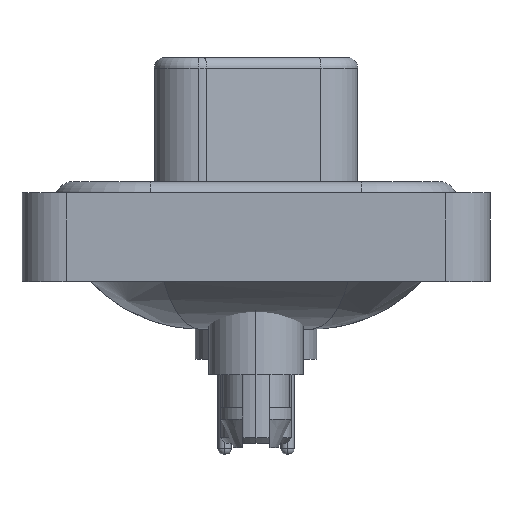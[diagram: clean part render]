
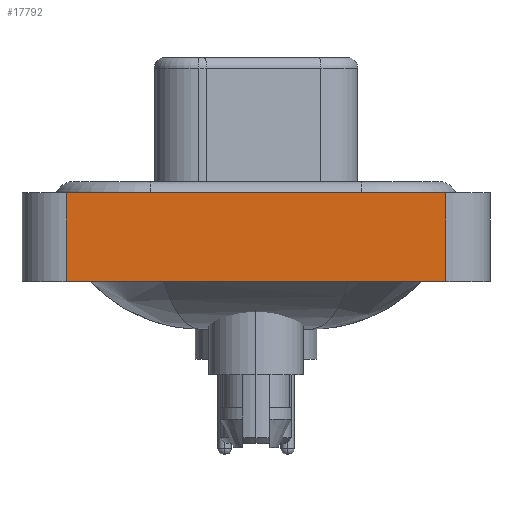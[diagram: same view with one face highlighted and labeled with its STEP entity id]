
A CAD part, left-side view. The second image highlights one B-rep face of the part: STEP entity #17792.
In plain terms, the highlighted planar face has unit normal (-1, 0, 0).
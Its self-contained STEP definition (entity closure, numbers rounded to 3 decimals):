
#251 = CARTESIAN_POINT ( 'NONE',  ( -7.3, -8.55, 0.4 ) ) ;
#439 = VECTOR ( 'NONE', #1418, 1000. ) ;
#1330 = CARTESIAN_POINT ( 'NONE',  ( -7.3, -8.55, -3.6 ) ) ;
#1418 = DIRECTION ( 'NONE',  ( 0., 0., 1. ) ) ;
#2074 = VERTEX_POINT ( 'NONE', #14540 ) ;
#2771 = VERTEX_POINT ( 'NONE', #16749 ) ;
#3270 = LINE ( 'NONE', #12254, #15598 ) ;
#3776 = ORIENTED_EDGE ( 'NONE', *, *, #15197, .F. ) ;
#3849 = DIRECTION ( 'NONE',  ( 0., -1., 0. ) ) ;
#4607 = DIRECTION ( 'NONE',  ( -1., 0., 0. ) ) ;
#4795 = FACE_OUTER_BOUND ( 'NONE', #4888, .T. ) ;
#4888 = EDGE_LOOP ( 'NONE', ( #9670, #6928, #3776, #19806 ) ) ;
#6472 = EDGE_CURVE ( 'NONE', #2074, #17091, #15144, .T. ) ;
#6928 = ORIENTED_EDGE ( 'NONE', *, *, #6472, .F. ) ;
#7524 = LINE ( 'NONE', #18316, #18497 ) ;
#9670 = ORIENTED_EDGE ( 'NONE', *, *, #12478, .T. ) ;
#10204 = VECTOR ( 'NONE', #3849, 1000. ) ;
#10463 = DIRECTION ( 'NONE',  ( 0., 0., 1. ) ) ;
#10513 = VERTEX_POINT ( 'NONE', #1330 ) ;
#10986 = PLANE ( 'NONE',  #13005 ) ;
#12254 = CARTESIAN_POINT ( 'NONE',  ( -7.3, -8.55, -3.6 ) ) ;
#12478 = EDGE_CURVE ( 'NONE', #10513, #17091, #7524, .T. ) ;
#13005 = AXIS2_PLACEMENT_3D ( 'NONE', #17206, #4607, #17308 ) ;
#14540 = CARTESIAN_POINT ( 'NONE',  ( -7.3, 8.55, 0.4 ) ) ;
#15144 = LINE ( 'NONE', #18110, #10204 ) ;
#15197 = EDGE_CURVE ( 'NONE', #2771, #2074, #15452, .T. ) ;
#15452 = LINE ( 'NONE', #18223, #439 ) ;
#15598 = VECTOR ( 'NONE', #15684, 1000. ) ;
#15684 = DIRECTION ( 'NONE',  ( 0., -1., 0. ) ) ;
#16749 = CARTESIAN_POINT ( 'NONE',  ( -7.3, 8.55, -3.6 ) ) ;
#17091 = VERTEX_POINT ( 'NONE', #251 ) ;
#17206 = CARTESIAN_POINT ( 'NONE',  ( -7.3, -8.55, -3.6 ) ) ;
#17308 = DIRECTION ( 'NONE',  ( 0., 0., 1. ) ) ;
#17792 = ADVANCED_FACE ( 'NONE', ( #4795 ), #10986, .T. ) ;
#17818 = EDGE_CURVE ( 'NONE', #2771, #10513, #3270, .T. ) ;
#18110 = CARTESIAN_POINT ( 'NONE',  ( -7.3, -8.55, 0.4 ) ) ;
#18223 = CARTESIAN_POINT ( 'NONE',  ( -7.3, 8.55, -3.6 ) ) ;
#18316 = CARTESIAN_POINT ( 'NONE',  ( -7.3, -8.55, -3.6 ) ) ;
#18497 = VECTOR ( 'NONE', #10463, 1000. ) ;
#19806 = ORIENTED_EDGE ( 'NONE', *, *, #17818, .T. ) ;
